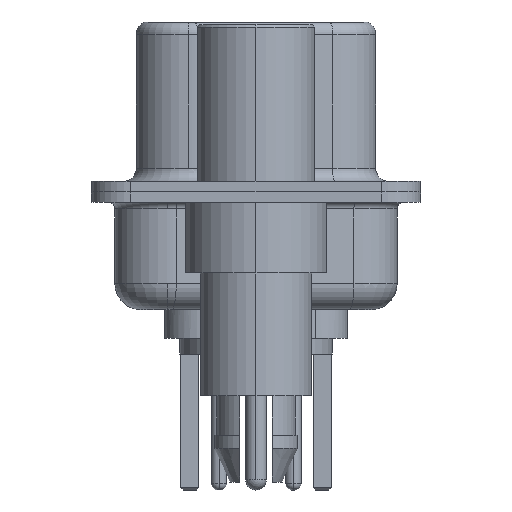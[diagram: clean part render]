
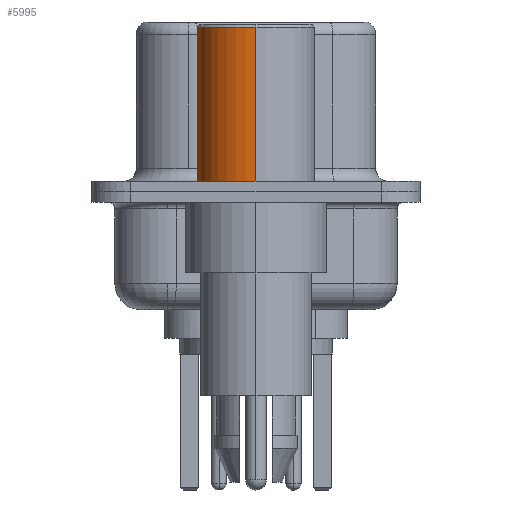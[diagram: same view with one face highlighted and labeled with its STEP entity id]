
A CAD part, left-side view. The second image highlights one B-rep face of the part: STEP entity #5995.
In plain terms, the highlighted cylindrical face has radius 2.25 mm (diameter 4.5 mm), a partial arc.
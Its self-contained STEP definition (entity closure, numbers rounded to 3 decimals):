
#721 = AXIS2_PLACEMENT_3D ( 'NONE', #19027, #11064, #5262 ) ;
#804 = CARTESIAN_POINT ( 'NONE',  ( -2.25, 0., 6.3 ) ) ;
#841 = ORIENTED_EDGE ( 'NONE', *, *, #9746, .F. ) ;
#3053 = AXIS2_PLACEMENT_3D ( 'NONE', #17977, #8087, #20046 ) ;
#3526 = CARTESIAN_POINT ( 'NONE',  ( -2.25, 0., 0.4 ) ) ;
#4497 = CARTESIAN_POINT ( 'NONE',  ( 2.25, 0., 0.4 ) ) ;
#5262 = DIRECTION ( 'NONE',  ( 1., 0., 0. ) ) ;
#5352 = VERTEX_POINT ( 'NONE', #3526 ) ;
#5995 = ADVANCED_FACE ( 'NONE', ( #15286 ), #6895, .T. ) ;
#6728 = VERTEX_POINT ( 'NONE', #9291 ) ;
#6855 = EDGE_LOOP ( 'NONE', ( #9431, #12546, #841, #19690 ) ) ;
#6895 = CYLINDRICAL_SURFACE ( 'NONE', #721, 2.25 ) ;
#8087 = DIRECTION ( 'NONE',  ( 0., 0., 1. ) ) ;
#9291 = CARTESIAN_POINT ( 'NONE',  ( 2.25, 0., 6.3 ) ) ;
#9431 = ORIENTED_EDGE ( 'NONE', *, *, #25377, .T. ) ;
#9746 = EDGE_CURVE ( 'NONE', #6728, #15730, #21460, .T. ) ;
#10259 = LINE ( 'NONE', #19753, #14930 ) ;
#10644 = DIRECTION ( 'NONE',  ( 1., 0., 0. ) ) ;
#11064 = DIRECTION ( 'NONE',  ( 0., 0., 1. ) ) ;
#11174 = DIRECTION ( 'NONE',  ( 0., 0., 1. ) ) ;
#12546 = ORIENTED_EDGE ( 'NONE', *, *, #23112, .T. ) ;
#12738 = DIRECTION ( 'NONE',  ( 0., 0., 1. ) ) ;
#12976 = CIRCLE ( 'NONE', #3053, 2.25 ) ;
#14930 = VECTOR ( 'NONE', #17870, 1000. ) ;
#15286 = FACE_OUTER_BOUND ( 'NONE', #6855, .T. ) ;
#15730 = VERTEX_POINT ( 'NONE', #804 ) ;
#17870 = DIRECTION ( 'NONE',  ( 0., 0., 1. ) ) ;
#17977 = CARTESIAN_POINT ( 'NONE',  ( 0., 0., 0.4 ) ) ;
#19027 = CARTESIAN_POINT ( 'NONE',  ( 0., 0., 0.581 ) ) ;
#19690 = ORIENTED_EDGE ( 'NONE', *, *, #20030, .F. ) ;
#19753 = CARTESIAN_POINT ( 'NONE',  ( 2.25, 0., 0.581 ) ) ;
#20030 = EDGE_CURVE ( 'NONE', #22116, #6728, #10259, .T. ) ;
#20046 = DIRECTION ( 'NONE',  ( 1., 0., 0. ) ) ;
#21311 = VECTOR ( 'NONE', #11174, 1000. ) ;
#21460 = CIRCLE ( 'NONE', #21529, 2.25 ) ;
#21529 = AXIS2_PLACEMENT_3D ( 'NONE', #24815, #12738, #10644 ) ;
#22116 = VERTEX_POINT ( 'NONE', #4497 ) ;
#23049 = CARTESIAN_POINT ( 'NONE',  ( -2.25, 0., 0.581 ) ) ;
#23112 = EDGE_CURVE ( 'NONE', #5352, #15730, #23460, .T. ) ;
#23460 = LINE ( 'NONE', #23049, #21311 ) ;
#24815 = CARTESIAN_POINT ( 'NONE',  ( 0., 0., 6.3 ) ) ;
#25377 = EDGE_CURVE ( 'NONE', #22116, #5352, #12976, .T. ) ;
